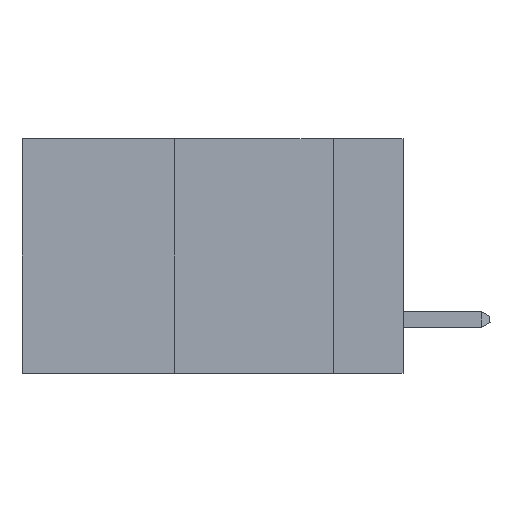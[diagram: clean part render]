
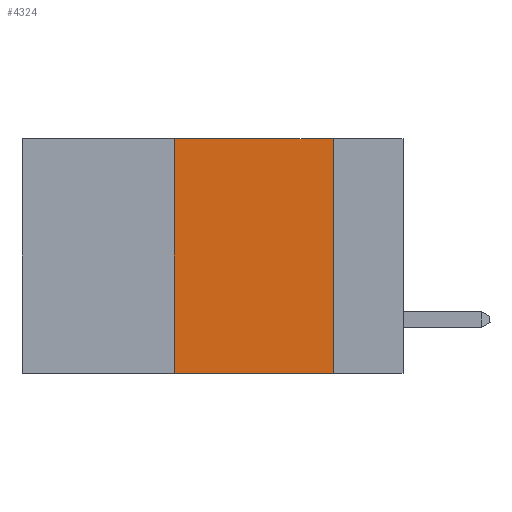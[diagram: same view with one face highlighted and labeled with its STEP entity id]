
A CAD part, left-side view. The second image highlights one B-rep face of the part: STEP entity #4324.
In plain terms, the highlighted planar face has unit normal (-1, 0, 0).
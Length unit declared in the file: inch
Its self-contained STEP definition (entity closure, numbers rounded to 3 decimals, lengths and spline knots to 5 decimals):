
#201 = DIRECTION ( 'NONE',  ( 0., -1., 0. ) ) ;
#367 = DIRECTION ( 'NONE',  ( 0., 0., 1. ) ) ;
#464 = LINE ( 'NONE', #9559, #5614 ) ;
#665 = VERTEX_POINT ( 'NONE', #12835 ) ;
#940 = EDGE_LOOP ( 'NONE', ( #8661, #10875, #1548, #9130 ) ) ;
#1413 = LINE ( 'NONE', #10827, #12086 ) ;
#1548 = ORIENTED_EDGE ( 'NONE', *, *, #12842, .F. ) ;
#2558 = DIRECTION ( 'NONE',  ( 0., -1., 0. ) ) ;
#2710 = LINE ( 'NONE', #10965, #7974 ) ;
#3058 = VERTEX_POINT ( 'NONE', #9856 ) ;
#4324 = ADVANCED_FACE ( 'NONE', ( #13018 ), #4393, .F. ) ;
#4393 = PLANE ( 'NONE',  #7587 ) ;
#5614 = VECTOR ( 'NONE', #2558, 39.37008 ) ;
#5914 = LINE ( 'NONE', #12489, #11942 ) ;
#6717 = VERTEX_POINT ( 'NONE', #12254 ) ;
#7587 = AXIS2_PLACEMENT_3D ( 'NONE', #12691, #7729, #9718 ) ;
#7729 = DIRECTION ( 'NONE',  ( 1., 0., 0. ) ) ;
#7974 = VECTOR ( 'NONE', #201, 39.37008 ) ;
#8661 = ORIENTED_EDGE ( 'NONE', *, *, #12141, .F. ) ;
#9130 = ORIENTED_EDGE ( 'NONE', *, *, #12287, .T. ) ;
#9559 = CARTESIAN_POINT ( 'NONE',  ( 0., 0.6, 0. ) ) ;
#9718 = DIRECTION ( 'NONE',  ( 0., 0., -1. ) ) ;
#9856 = CARTESIAN_POINT ( 'NONE',  ( 0., 0.36, -0.37 ) ) ;
#9991 = CARTESIAN_POINT ( 'NONE',  ( 0., 0.11, -0.37 ) ) ;
#10827 = CARTESIAN_POINT ( 'NONE',  ( 0., 0.11, 0. ) ) ;
#10875 = ORIENTED_EDGE ( 'NONE', *, *, #11695, .F. ) ;
#10965 = CARTESIAN_POINT ( 'NONE',  ( 0., 0.6, -0.37 ) ) ;
#11559 = VERTEX_POINT ( 'NONE', #9991 ) ;
#11695 = EDGE_CURVE ( 'NONE', #665, #6717, #464, .T. ) ;
#11942 = VECTOR ( 'NONE', #367, 39.37008 ) ;
#12086 = VECTOR ( 'NONE', #12862, 39.37008 ) ;
#12141 = EDGE_CURVE ( 'NONE', #6717, #11559, #1413, .T. ) ;
#12254 = CARTESIAN_POINT ( 'NONE',  ( 0., 0.11, 0. ) ) ;
#12287 = EDGE_CURVE ( 'NONE', #3058, #11559, #2710, .T. ) ;
#12489 = CARTESIAN_POINT ( 'NONE',  ( 0., 0.36, 0. ) ) ;
#12691 = CARTESIAN_POINT ( 'NONE',  ( 0., 0.6, 0. ) ) ;
#12835 = CARTESIAN_POINT ( 'NONE',  ( 0., 0.36, 0. ) ) ;
#12842 = EDGE_CURVE ( 'NONE', #3058, #665, #5914, .T. ) ;
#12862 = DIRECTION ( 'NONE',  ( 0., 0., -1. ) ) ;
#13018 = FACE_OUTER_BOUND ( 'NONE', #940, .T. ) ;
